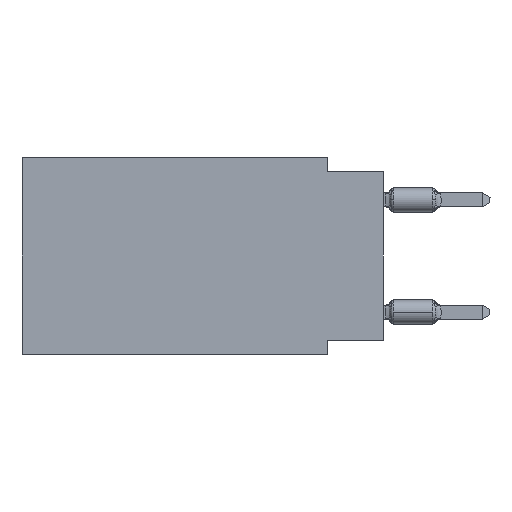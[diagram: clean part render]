
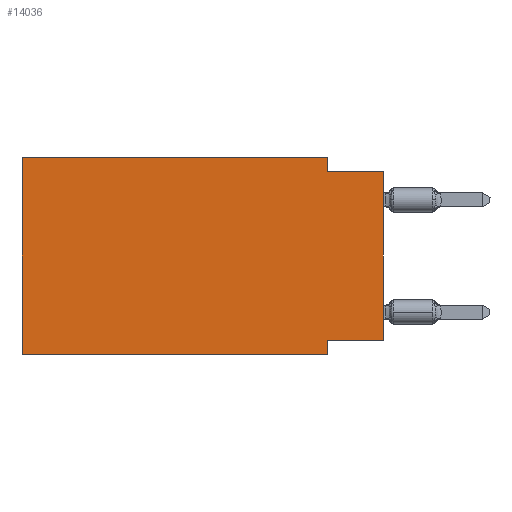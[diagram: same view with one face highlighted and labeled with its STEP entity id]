
A CAD part, left-side view. The second image highlights one B-rep face of the part: STEP entity #14036.
In plain terms, the highlighted planar face has unit normal (-1, 0, 0).
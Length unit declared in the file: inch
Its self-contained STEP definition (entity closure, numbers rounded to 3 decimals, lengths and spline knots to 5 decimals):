
#661 = AXIS2_PLACEMENT_3D ( 'NONE', #14312, #3900, #22900 ) ;
#1389 = EDGE_CURVE ( 'NONE', #26729, #9723, #10554, .T. ) ;
#2058 = FACE_OUTER_BOUND ( 'NONE', #15501, .T. ) ;
#2397 = DIRECTION ( 'NONE',  ( 0., 0., -1. ) ) ;
#2518 = VECTOR ( 'NONE', #14318, 39.37008 ) ;
#2744 = LINE ( 'NONE', #9494, #10847 ) ;
#2924 = CARTESIAN_POINT ( 'NONE',  ( 0., 0.645, -0.35 ) ) ;
#3014 = DIRECTION ( 'NONE',  ( 0., 0., -1. ) ) ;
#3327 = VECTOR ( 'NONE', #2397, 39.37008 ) ;
#3900 = DIRECTION ( 'NONE',  ( 1., 0., 0. ) ) ;
#4367 = LINE ( 'NONE', #26198, #8276 ) ;
#5318 = LINE ( 'NONE', #17982, #6381 ) ;
#5473 = ORIENTED_EDGE ( 'NONE', *, *, #5635, .F. ) ;
#5574 = EDGE_CURVE ( 'NONE', #21678, #14189, #4367, .T. ) ;
#5635 = EDGE_CURVE ( 'NONE', #9723, #21678, #17597, .T. ) ;
#6047 = CARTESIAN_POINT ( 'NONE',  ( 0., 0.645, 0. ) ) ;
#6089 = ORIENTED_EDGE ( 'NONE', *, *, #17914, .F. ) ;
#6381 = VECTOR ( 'NONE', #16429, 39.37008 ) ;
#7099 = EDGE_CURVE ( 'NONE', #13641, #14189, #27047, .T. ) ;
#7892 = CARTESIAN_POINT ( 'NONE',  ( 0., 0., 0. ) ) ;
#8017 = CARTESIAN_POINT ( 'NONE',  ( 0., 0., -0.325 ) ) ;
#8276 = VECTOR ( 'NONE', #15343, 39.37008 ) ;
#8506 = ORIENTED_EDGE ( 'NONE', *, *, #22960, .F. ) ;
#8946 = CARTESIAN_POINT ( 'NONE',  ( 0., 0.1, 0. ) ) ;
#9406 = CARTESIAN_POINT ( 'NONE',  ( 0., 0.645, -0.35 ) ) ;
#9494 = CARTESIAN_POINT ( 'NONE',  ( 0., 0.1, -0.35 ) ) ;
#9673 = ORIENTED_EDGE ( 'NONE', *, *, #5574, .F. ) ;
#9723 = VERTEX_POINT ( 'NONE', #8946 ) ;
#10281 = VECTOR ( 'NONE', #12519, 39.37008 ) ;
#10554 = LINE ( 'NONE', #6047, #10281 ) ;
#10595 = ORIENTED_EDGE ( 'NONE', *, *, #22190, .F. ) ;
#10847 = VECTOR ( 'NONE', #3014, 39.37008 ) ;
#10902 = ORIENTED_EDGE ( 'NONE', *, *, #1389, .F. ) ;
#11637 = DIRECTION ( 'NONE',  ( 0., -1., 0. ) ) ;
#11722 = ORIENTED_EDGE ( 'NONE', *, *, #7099, .T. ) ;
#11946 = ORIENTED_EDGE ( 'NONE', *, *, #27005, .T. ) ;
#12519 = DIRECTION ( 'NONE',  ( 0., -1., 0. ) ) ;
#13641 = VERTEX_POINT ( 'NONE', #8017 ) ;
#14036 = ADVANCED_FACE ( 'NONE', ( #2058 ), #23179, .F. ) ;
#14189 = VERTEX_POINT ( 'NONE', #26282 ) ;
#14199 = CARTESIAN_POINT ( 'NONE',  ( 0., 0.645, 0. ) ) ;
#14312 = CARTESIAN_POINT ( 'NONE',  ( 0., 0.645, 0. ) ) ;
#14318 = DIRECTION ( 'NONE',  ( 0., 1., 0. ) ) ;
#15343 = DIRECTION ( 'NONE',  ( 0., -1., 0. ) ) ;
#15501 = EDGE_LOOP ( 'NONE', ( #11722, #9673, #5473, #10902, #8506, #11946, #10595, #6089 ) ) ;
#16429 = DIRECTION ( 'NONE',  ( 0., 0., 1. ) ) ;
#17555 = CARTESIAN_POINT ( 'NONE',  ( 0., 0.1, -0.325 ) ) ;
#17597 = LINE ( 'NONE', #19430, #3327 ) ;
#17810 = VERTEX_POINT ( 'NONE', #26593 ) ;
#17820 = CARTESIAN_POINT ( 'NONE',  ( 0., 0.1, -0.025 ) ) ;
#17836 = VERTEX_POINT ( 'NONE', #9406 ) ;
#17914 = EDGE_CURVE ( 'NONE', #13641, #18546, #22903, .T. ) ;
#17982 = CARTESIAN_POINT ( 'NONE',  ( 0., 0.645, 0. ) ) ;
#18396 = VECTOR ( 'NONE', #22663, 39.37008 ) ;
#18546 = VERTEX_POINT ( 'NONE', #17555 ) ;
#19430 = CARTESIAN_POINT ( 'NONE',  ( 0., 0.1, 0. ) ) ;
#20214 = VECTOR ( 'NONE', #11637, 39.37008 ) ;
#21678 = VERTEX_POINT ( 'NONE', #17820 ) ;
#22190 = EDGE_CURVE ( 'NONE', #18546, #17810, #2744, .T. ) ;
#22663 = DIRECTION ( 'NONE',  ( 0., 0., 1. ) ) ;
#22900 = DIRECTION ( 'NONE',  ( 0., 0., -1. ) ) ;
#22903 = LINE ( 'NONE', #25035, #2518 ) ;
#22960 = EDGE_CURVE ( 'NONE', #17836, #26729, #5318, .T. ) ;
#23179 = PLANE ( 'NONE',  #661 ) ;
#24321 = LINE ( 'NONE', #2924, #20214 ) ;
#25035 = CARTESIAN_POINT ( 'NONE',  ( 0., 0., -0.325 ) ) ;
#26198 = CARTESIAN_POINT ( 'NONE',  ( 0., 0., -0.025 ) ) ;
#26282 = CARTESIAN_POINT ( 'NONE',  ( 0., 0., -0.025 ) ) ;
#26593 = CARTESIAN_POINT ( 'NONE',  ( 0., 0.1, -0.35 ) ) ;
#26729 = VERTEX_POINT ( 'NONE', #14199 ) ;
#27005 = EDGE_CURVE ( 'NONE', #17836, #17810, #24321, .T. ) ;
#27047 = LINE ( 'NONE', #7892, #18396 ) ;
